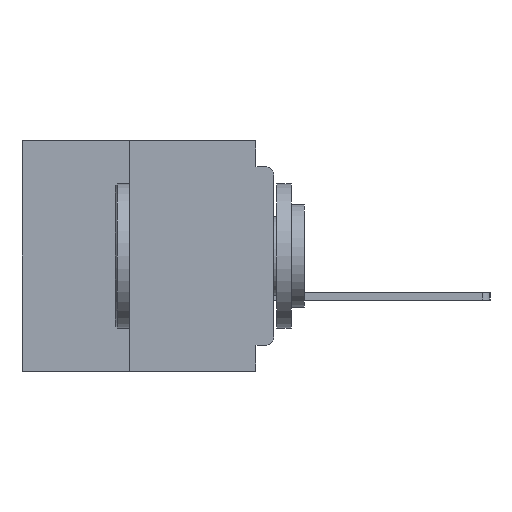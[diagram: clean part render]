
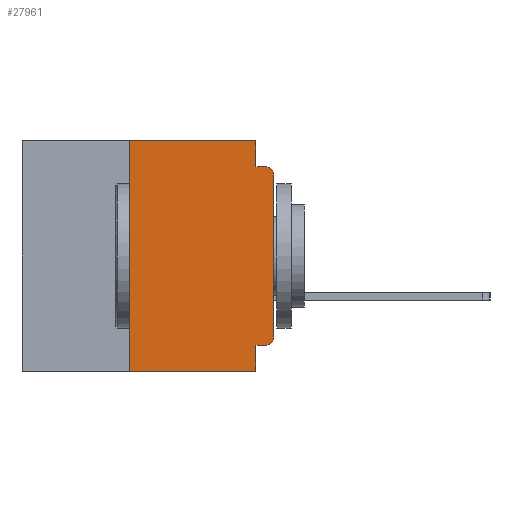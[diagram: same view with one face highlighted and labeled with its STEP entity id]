
A CAD part, left-side view. The second image highlights one B-rep face of the part: STEP entity #27961.
In plain terms, the highlighted planar face has unit normal (-1, 0, 0).
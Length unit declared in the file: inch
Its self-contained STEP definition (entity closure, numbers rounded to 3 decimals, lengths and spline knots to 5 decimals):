
#154 = DIRECTION ( 'NONE',  ( 1., 0., 0. ) ) ;
#400 = DIRECTION ( 'NONE',  ( 0., -1., 0. ) ) ;
#458 = LINE ( 'NONE', #3473, #16697 ) ;
#1896 = EDGE_CURVE ( 'NONE', #25886, #28039, #5293, .T. ) ;
#2047 = CIRCLE ( 'NONE', #9371, 0.015 ) ;
#2930 = ORIENTED_EDGE ( 'NONE', *, *, #14761, .F. ) ;
#3177 = LINE ( 'NONE', #11786, #25131 ) ;
#3473 = CARTESIAN_POINT ( 'NONE',  ( 0., 0.031, 0. ) ) ;
#3600 = DIRECTION ( 'NONE',  ( 0., 0., -1. ) ) ;
#3968 = EDGE_CURVE ( 'NONE', #15260, #23717, #20859, .T. ) ;
#4086 = ORIENTED_EDGE ( 'NONE', *, *, #1896, .T. ) ;
#4950 = ORIENTED_EDGE ( 'NONE', *, *, #19142, .T. ) ;
#5293 = CIRCLE ( 'NONE', #33268, 0.015 ) ;
#5803 = CARTESIAN_POINT ( 'NONE',  ( 0., 0., -0.06 ) ) ;
#5884 = LINE ( 'NONE', #14173, #20231 ) ;
#6782 = CARTESIAN_POINT ( 'NONE',  ( 0., 0.25, 0. ) ) ;
#7655 = CARTESIAN_POINT ( 'NONE',  ( 0., 0., -0.355 ) ) ;
#8314 = LINE ( 'NONE', #10948, #30128 ) ;
#9220 = DIRECTION ( 'NONE',  ( 0., 0., -1. ) ) ;
#9334 = EDGE_CURVE ( 'NONE', #22347, #28039, #19017, .T. ) ;
#9371 = AXIS2_PLACEMENT_3D ( 'NONE', #26775, #9698, #29597 ) ;
#9670 = EDGE_CURVE ( 'NONE', #36776, #26212, #28296, .T. ) ;
#9698 = DIRECTION ( 'NONE',  ( -1., 0., 0. ) ) ;
#10163 = DIRECTION ( 'NONE',  ( 0., -1., 0. ) ) ;
#10475 = ORIENTED_EDGE ( 'NONE', *, *, #14667, .F. ) ;
#10515 = VECTOR ( 'NONE', #13147, 39.37008 ) ;
#10948 = CARTESIAN_POINT ( 'NONE',  ( 0., 0., 0. ) ) ;
#11139 = DIRECTION ( 'NONE',  ( -1., 0., 0. ) ) ;
#11299 = DIRECTION ( 'NONE',  ( 0., 0., -1. ) ) ;
#11786 = CARTESIAN_POINT ( 'NONE',  ( 0., 0.25, -0.4 ) ) ;
#12028 = VERTEX_POINT ( 'NONE', #34285 ) ;
#13147 = DIRECTION ( 'NONE',  ( 0., -1., 0. ) ) ;
#13843 = VECTOR ( 'NONE', #24763, 39.37008 ) ;
#14168 = EDGE_CURVE ( 'NONE', #36472, #12028, #2047, .T. ) ;
#14173 = CARTESIAN_POINT ( 'NONE',  ( 0., 0.031, -0.4 ) ) ;
#14667 = EDGE_CURVE ( 'NONE', #36776, #15260, #3177, .T. ) ;
#14761 = EDGE_CURVE ( 'NONE', #23717, #22347, #458, .T. ) ;
#15029 = EDGE_CURVE ( 'NONE', #23315, #26212, #5884, .T. ) ;
#15136 = CARTESIAN_POINT ( 'NONE',  ( 0., 0.031, -0.4 ) ) ;
#15260 = VERTEX_POINT ( 'NONE', #6782 ) ;
#15385 = CARTESIAN_POINT ( 'NONE',  ( 0., 0.015, -0.045 ) ) ;
#15855 = CARTESIAN_POINT ( 'NONE',  ( 0., 0.031, 0. ) ) ;
#15906 = CARTESIAN_POINT ( 'NONE',  ( 0., 0., -0.045 ) ) ;
#16697 = VECTOR ( 'NONE', #3600, 39.37008 ) ;
#17143 = CARTESIAN_POINT ( 'NONE',  ( 0., 0.031, -0.045 ) ) ;
#17252 = EDGE_CURVE ( 'NONE', #36472, #23315, #21440, .T. ) ;
#17413 = PLANE ( 'NONE',  #21027 ) ;
#18853 = EDGE_LOOP ( 'NONE', ( #4950, #4086, #27853, #2930, #33506, #10475, #23978, #24585, #30972, #20225 ) ) ;
#19017 = LINE ( 'NONE', #15906, #10515 ) ;
#19142 = EDGE_CURVE ( 'NONE', #12028, #25886, #8314, .T. ) ;
#19237 = FACE_OUTER_BOUND ( 'NONE', #18853, .T. ) ;
#19302 = CARTESIAN_POINT ( 'NONE',  ( 0., 0.031, -0.355 ) ) ;
#20225 = ORIENTED_EDGE ( 'NONE', *, *, #14168, .T. ) ;
#20231 = VECTOR ( 'NONE', #11299, 39.37008 ) ;
#20275 = DIRECTION ( 'NONE',  ( 0., 0., -1. ) ) ;
#20787 = VECTOR ( 'NONE', #400, 39.37008 ) ;
#20859 = LINE ( 'NONE', #27215, #22637 ) ;
#21027 = AXIS2_PLACEMENT_3D ( 'NONE', #34329, #154, #20275 ) ;
#21440 = LINE ( 'NONE', #7655, #13843 ) ;
#22347 = VERTEX_POINT ( 'NONE', #17143 ) ;
#22637 = VECTOR ( 'NONE', #10163, 39.37008 ) ;
#23288 = DIRECTION ( 'NONE',  ( 0., 0., 1. ) ) ;
#23315 = VERTEX_POINT ( 'NONE', #19302 ) ;
#23717 = VERTEX_POINT ( 'NONE', #15855 ) ;
#23764 = CARTESIAN_POINT ( 'NONE',  ( 0., 0.015, -0.355 ) ) ;
#23978 = ORIENTED_EDGE ( 'NONE', *, *, #9670, .T. ) ;
#24585 = ORIENTED_EDGE ( 'NONE', *, *, #15029, .F. ) ;
#24763 = DIRECTION ( 'NONE',  ( 0., 1., 0. ) ) ;
#25131 = VECTOR ( 'NONE', #23288, 39.37008 ) ;
#25886 = VERTEX_POINT ( 'NONE', #5803 ) ;
#26212 = VERTEX_POINT ( 'NONE', #15136 ) ;
#26775 = CARTESIAN_POINT ( 'NONE',  ( 0., 0.015, -0.34 ) ) ;
#27215 = CARTESIAN_POINT ( 'NONE',  ( 0., 0.437, 0. ) ) ;
#27853 = ORIENTED_EDGE ( 'NONE', *, *, #9334, .F. ) ;
#27928 = CARTESIAN_POINT ( 'NONE',  ( 0., 0.25, -0.4 ) ) ;
#27961 = ADVANCED_FACE ( 'NONE', ( #19237 ), #17413, .F. ) ;
#28039 = VERTEX_POINT ( 'NONE', #15385 ) ;
#28296 = LINE ( 'NONE', #34566, #20787 ) ;
#29597 = DIRECTION ( 'NONE',  ( 0., 0., -1. ) ) ;
#30128 = VECTOR ( 'NONE', #30841, 39.37008 ) ;
#30841 = DIRECTION ( 'NONE',  ( 0., 0., 1. ) ) ;
#30972 = ORIENTED_EDGE ( 'NONE', *, *, #17252, .F. ) ;
#32624 = CARTESIAN_POINT ( 'NONE',  ( 0., 0.015, -0.06 ) ) ;
#33268 = AXIS2_PLACEMENT_3D ( 'NONE', #32624, #11139, #9220 ) ;
#33506 = ORIENTED_EDGE ( 'NONE', *, *, #3968, .F. ) ;
#34285 = CARTESIAN_POINT ( 'NONE',  ( 0., 0., -0.34 ) ) ;
#34329 = CARTESIAN_POINT ( 'NONE',  ( 0., 0.437, 0. ) ) ;
#34566 = CARTESIAN_POINT ( 'NONE',  ( 0., 0.437, -0.4 ) ) ;
#36472 = VERTEX_POINT ( 'NONE', #23764 ) ;
#36776 = VERTEX_POINT ( 'NONE', #27928 ) ;
